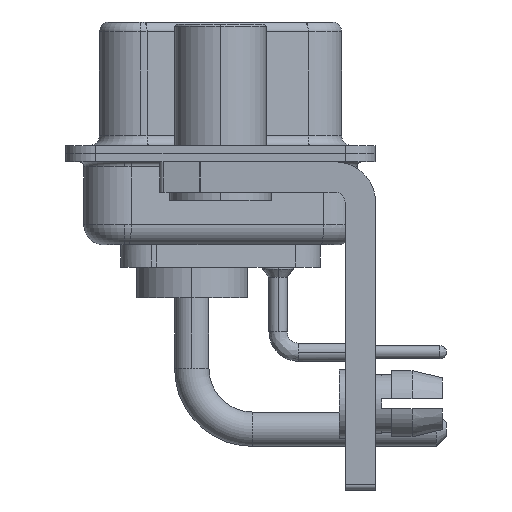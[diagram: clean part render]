
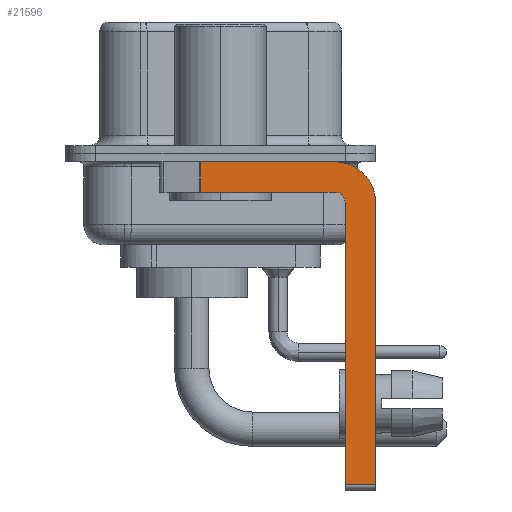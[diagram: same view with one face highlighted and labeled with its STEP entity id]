
A CAD part, left-side view. The second image highlights one B-rep face of the part: STEP entity #21596.
In plain terms, the highlighted planar face has unit normal (-1, 0, 0).
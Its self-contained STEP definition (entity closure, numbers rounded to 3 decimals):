
#198 = PLANE ( 'NONE',  #10553 ) ;
#477 = VERTEX_POINT ( 'NONE', #26135 ) ;
#1273 = EDGE_CURVE ( 'NONE', #21546, #12501, #24029, .T. ) ;
#1716 = VERTEX_POINT ( 'NONE', #10397 ) ;
#1789 = CARTESIAN_POINT ( 'NONE',  ( -2.9, -6.15, -16.6 ) ) ;
#2340 = CIRCLE ( 'NONE', #22277, 0.5 ) ;
#2883 = ORIENTED_EDGE ( 'NONE', *, *, #15856, .F. ) ;
#3198 = EDGE_CURVE ( 'NONE', #4140, #4945, #4117, .T. ) ;
#3501 = LINE ( 'NONE', #27061, #23056 ) ;
#3559 = DIRECTION ( 'NONE',  ( 1., 0., 0. ) ) ;
#4099 = LINE ( 'NONE', #15596, #10570 ) ;
#4117 = LINE ( 'NONE', #14482, #9276 ) ;
#4140 = VERTEX_POINT ( 'NONE', #4442 ) ;
#4442 = CARTESIAN_POINT ( 'NONE',  ( -2.9, 0.978, -0.4 ) ) ;
#4506 = EDGE_CURVE ( 'NONE', #22500, #1716, #16630, .T. ) ;
#4945 = VERTEX_POINT ( 'NONE', #21113 ) ;
#5563 = VECTOR ( 'NONE', #25319, 1000. ) ;
#5770 = ORIENTED_EDGE ( 'NONE', *, *, #27357, .F. ) ;
#5837 = DIRECTION ( 'NONE',  ( 0., 0., -1. ) ) ;
#5887 = EDGE_CURVE ( 'NONE', #14152, #4945, #27437, .T. ) ;
#6313 = DIRECTION ( 'NONE',  ( 0., 0., 1. ) ) ;
#7628 = CARTESIAN_POINT ( 'NONE',  ( -2.9, -5.65, -2.4 ) ) ;
#7997 = CARTESIAN_POINT ( 'NONE',  ( -2.9, -5.65, -1.9 ) ) ;
#8251 = VECTOR ( 'NONE', #5837, 1000. ) ;
#9276 = VECTOR ( 'NONE', #18749, 1000. ) ;
#10192 = CIRCLE ( 'NONE', #26892, 2. ) ;
#10397 = CARTESIAN_POINT ( 'NONE',  ( -2.9, -7.65, -16.35 ) ) ;
#10553 = AXIS2_PLACEMENT_3D ( 'NONE', #25734, #14940, #23596 ) ;
#10570 = VECTOR ( 'NONE', #13320, 1000. ) ;
#11084 = ORIENTED_EDGE ( 'NONE', *, *, #5887, .F. ) ;
#12501 = VERTEX_POINT ( 'NONE', #16417 ) ;
#13320 = DIRECTION ( 'NONE',  ( 0., -1., 0. ) ) ;
#14152 = VERTEX_POINT ( 'NONE', #19792 ) ;
#14482 = CARTESIAN_POINT ( 'NONE',  ( -2.9, 0.978, -1.9 ) ) ;
#14559 = DIRECTION ( 'NONE',  ( 0., -1., 0. ) ) ;
#14799 = CARTESIAN_POINT ( 'NONE',  ( -2.9, -6.15, -16.35 ) ) ;
#14940 = DIRECTION ( 'NONE',  ( 1., 0., 0. ) ) ;
#15494 = ORIENTED_EDGE ( 'NONE', *, *, #4506, .F. ) ;
#15596 = CARTESIAN_POINT ( 'NONE',  ( -2.9, 3., -0.4 ) ) ;
#15856 = EDGE_CURVE ( 'NONE', #4140, #477, #4099, .T. ) ;
#16417 = CARTESIAN_POINT ( 'NONE',  ( -2.9, -6.15, -2.4 ) ) ;
#16630 = LINE ( 'NONE', #19032, #8251 ) ;
#16647 = ORIENTED_EDGE ( 'NONE', *, *, #22848, .T. ) ;
#17383 = ORIENTED_EDGE ( 'NONE', *, *, #3198, .T. ) ;
#17559 = EDGE_CURVE ( 'NONE', #477, #22500, #10192, .T. ) ;
#18749 = DIRECTION ( 'NONE',  ( 0., 0., -1. ) ) ;
#19032 = CARTESIAN_POINT ( 'NONE',  ( -2.9, -7.65, -2.4 ) ) ;
#19372 = EDGE_LOOP ( 'NONE', ( #2883, #17383, #11084, #5770, #26687, #16647, #15494, #21551 ) ) ;
#19792 = CARTESIAN_POINT ( 'NONE',  ( -2.9, -5.65, -1.9 ) ) ;
#21113 = CARTESIAN_POINT ( 'NONE',  ( -2.9, 0.978, -1.9 ) ) ;
#21452 = FACE_OUTER_BOUND ( 'NONE', #19372, .T. ) ;
#21532 = CARTESIAN_POINT ( 'NONE',  ( -2.9, -7.65, -2.4 ) ) ;
#21546 = VERTEX_POINT ( 'NONE', #14799 ) ;
#21551 = ORIENTED_EDGE ( 'NONE', *, *, #17559, .F. ) ;
#21596 = ADVANCED_FACE ( 'NONE', ( #21452 ), #198, .F. ) ;
#22277 = AXIS2_PLACEMENT_3D ( 'NONE', #7628, #22686, #24943 ) ;
#22500 = VERTEX_POINT ( 'NONE', #21532 ) ;
#22686 = DIRECTION ( 'NONE',  ( -1., 0., 0. ) ) ;
#22848 = EDGE_CURVE ( 'NONE', #21546, #1716, #3501, .T. ) ;
#22875 = VECTOR ( 'NONE', #6313, 1000. ) ;
#23007 = CARTESIAN_POINT ( 'NONE',  ( -2.9, -5.65, -2.4 ) ) ;
#23056 = VECTOR ( 'NONE', #14559, 1000. ) ;
#23286 = DIRECTION ( 'NONE',  ( 0., 0., -1. ) ) ;
#23596 = DIRECTION ( 'NONE',  ( 0., 0., -1. ) ) ;
#24029 = LINE ( 'NONE', #1789, #22875 ) ;
#24943 = DIRECTION ( 'NONE',  ( 0., 0., 1. ) ) ;
#25319 = DIRECTION ( 'NONE',  ( 0., 1., 0. ) ) ;
#25734 = CARTESIAN_POINT ( 'NONE',  ( -2.9, -5.65, -2.4 ) ) ;
#26135 = CARTESIAN_POINT ( 'NONE',  ( -2.9, -5.65, -0.4 ) ) ;
#26687 = ORIENTED_EDGE ( 'NONE', *, *, #1273, .F. ) ;
#26892 = AXIS2_PLACEMENT_3D ( 'NONE', #23007, #3559, #23286 ) ;
#27061 = CARTESIAN_POINT ( 'NONE',  ( -2.9, -5.65, -16.35 ) ) ;
#27357 = EDGE_CURVE ( 'NONE', #12501, #14152, #2340, .T. ) ;
#27437 = LINE ( 'NONE', #7997, #5563 ) ;
